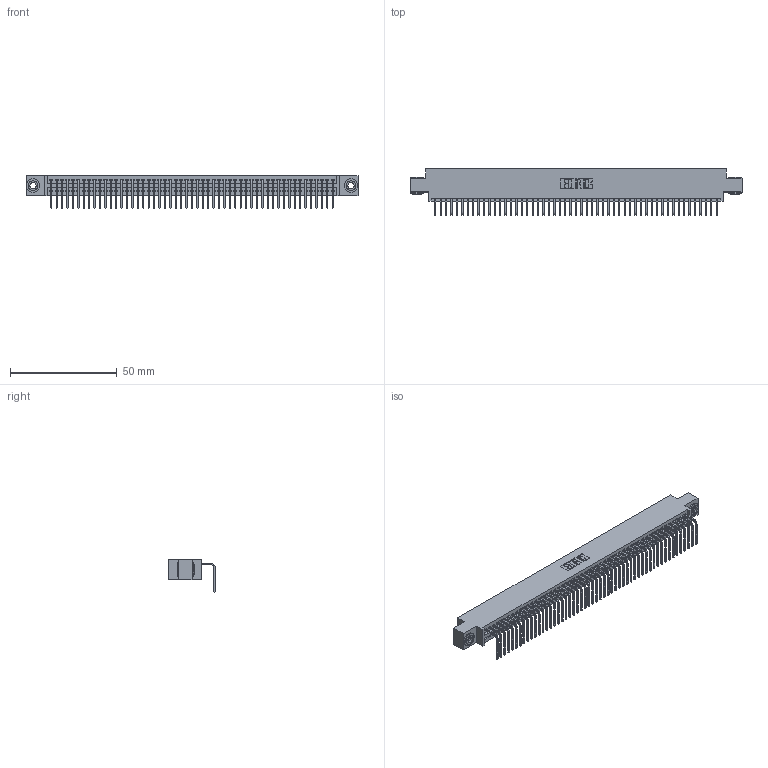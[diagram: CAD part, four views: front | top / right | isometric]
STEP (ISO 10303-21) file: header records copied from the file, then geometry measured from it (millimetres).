
FILE_DESCRIPTION (( 'STEP AP203' ), '1' );
FILE_NAME ('395-053-558-603.STEP', '2018-11-21T05:30:26', ( '' ), ( '' ), 'SwSTEP 2.0', 'SolidWorks 2016', '' );
FILE_SCHEMA (( 'CONFIG_CONTROL_DESIGN' ));
Length unit declared in the file: inch
Products named in the file (4): 345 Part_0.170 Offset - 0.156 Dia-TH; 345-292-001_558 Tail - 2; 345-250-002_345-250-002-102; 395-053-558-603
Assembly tree (56 placements, depth 2):
  395-053-558-603
    345 Part_0.170 Offset - 0.156 Dia-TH
    345-292-001_558 Tail - 2  x53
    345-250-002_345-250-002-102  x2
Bounding box: 155.83 x 21.83 x 15.37 mm (x, y, z)
Volume: 14973.5 mm3; surface area: 21426.6 mm2
Topology: 56 solids, 56 shells, 3348 faces, 10075 edges, 6642 vertices
Faces by surface type: plane 2320, cylinder 1020, cone 8
Entity records: 39274 total; most frequent: CARTESIAN_POINT 6782, ORIENTED_EDGE 6762, DIRECTION 5937, EDGE_CURVE 3381, VECTOR 3013, LINE 3013, VERTEX_POINT 2250, AXIS2_PLACEMENT_3D 1462
